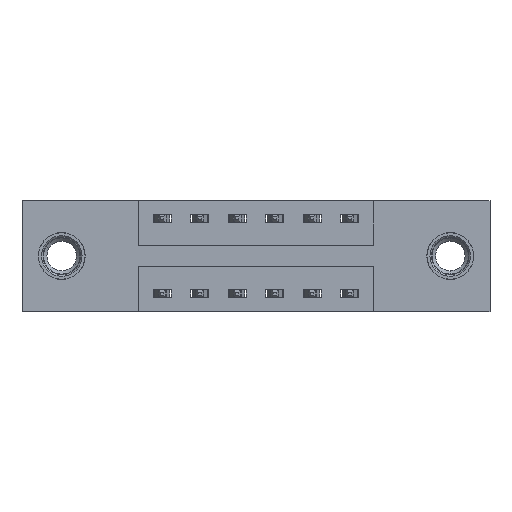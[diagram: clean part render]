
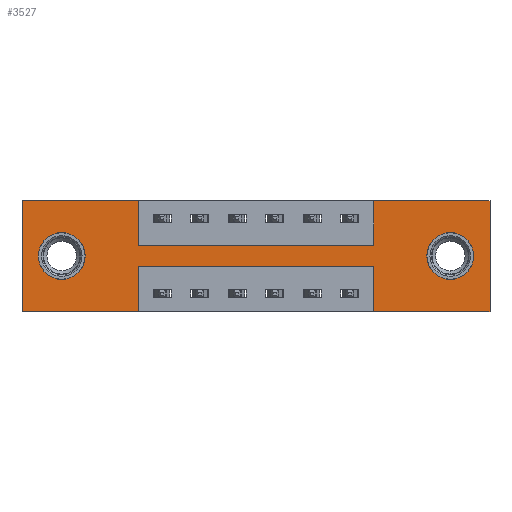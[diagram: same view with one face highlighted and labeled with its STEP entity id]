
A CAD part, front view. The second image highlights one B-rep face of the part: STEP entity #3527.
In plain terms, the highlighted planar face has unit normal (0, -1, 0).
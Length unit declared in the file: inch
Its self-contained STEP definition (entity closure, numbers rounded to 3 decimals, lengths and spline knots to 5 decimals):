
#77 = VECTOR ( 'NONE', #1908, 39.37008 ) ;
#117 = DIRECTION ( 'NONE',  ( 0., 0., -1. ) ) ;
#195 = DIRECTION ( 'NONE',  ( 0., 0., 1. ) ) ;
#220 = DIRECTION ( 'NONE',  ( -1., 0., 0. ) ) ;
#312 = AXIS2_PLACEMENT_3D ( 'NONE', #3044, #5407, #547 ) ;
#351 = CIRCLE ( 'NONE', #3444, 0.078 ) ;
#493 = CARTESIAN_POINT ( 'NONE',  ( 0.3875, 0., -0.22 ) ) ;
#547 = DIRECTION ( 'NONE',  ( 0., 0., -1. ) ) ;
#624 = DIRECTION ( 'NONE',  ( 0., 0., -1. ) ) ;
#731 = EDGE_CURVE ( 'NONE', #2609, #8651, #817, .T. ) ;
#736 = VECTOR ( 'NONE', #195, 39.37008 ) ;
#804 = AXIS2_PLACEMENT_3D ( 'NONE', #1364, #8633, #4704 ) ;
#805 = VECTOR ( 'NONE', #845, 39.37008 ) ;
#817 = CIRCLE ( 'NONE', #7860, 0.078 ) ;
#823 = FACE_OUTER_BOUND ( 'NONE', #9699, .T. ) ;
#845 = DIRECTION ( 'NONE',  ( -1., 0., 0. ) ) ;
#848 = CARTESIAN_POINT ( 'NONE',  ( 0., 0., -0.37 ) ) ;
#890 = ORIENTED_EDGE ( 'NONE', *, *, #5757, .F. ) ;
#955 = ORIENTED_EDGE ( 'NONE', *, *, #1147, .F. ) ;
#975 = DIRECTION ( 'NONE',  ( 0., 0., -1. ) ) ;
#1002 = CARTESIAN_POINT ( 'NONE',  ( 1.56, 0., 0. ) ) ;
#1065 = DIRECTION ( 'NONE',  ( 0., 0., 1. ) ) ;
#1078 = FACE_BOUND ( 'NONE', #9427, .T. ) ;
#1147 = EDGE_CURVE ( 'NONE', #9044, #2476, #7146, .T. ) ;
#1261 = VERTEX_POINT ( 'NONE', #493 ) ;
#1279 = CARTESIAN_POINT ( 'NONE',  ( 0.3875, 0., 0. ) ) ;
#1359 = DIRECTION ( 'NONE',  ( 1., 0., 0. ) ) ;
#1364 = CARTESIAN_POINT ( 'NONE',  ( 0.1325, 0., -0.185 ) ) ;
#1389 = CARTESIAN_POINT ( 'NONE',  ( 0.3875, 0., -0.37 ) ) ;
#1631 = EDGE_CURVE ( 'NONE', #7315, #5923, #5667, .T. ) ;
#1807 = CARTESIAN_POINT ( 'NONE',  ( 0., 0., 0. ) ) ;
#1809 = CARTESIAN_POINT ( 'NONE',  ( 0.1325, 0., -0.107 ) ) ;
#1888 = VECTOR ( 'NONE', #3370, 39.37008 ) ;
#1908 = DIRECTION ( 'NONE',  ( 1., 0., 0. ) ) ;
#1944 = ORIENTED_EDGE ( 'NONE', *, *, #7622, .F. ) ;
#2019 = CIRCLE ( 'NONE', #7383, 0.078 ) ;
#2164 = LINE ( 'NONE', #2536, #1888 ) ;
#2206 = ORIENTED_EDGE ( 'NONE', *, *, #5881, .F. ) ;
#2476 = VERTEX_POINT ( 'NONE', #9174 ) ;
#2500 = CARTESIAN_POINT ( 'NONE',  ( 1.4275, 0., -0.263 ) ) ;
#2536 = CARTESIAN_POINT ( 'NONE',  ( 1.1725, 0., 0. ) ) ;
#2582 = CARTESIAN_POINT ( 'NONE',  ( 0.3875, 0., -0.37 ) ) ;
#2609 = VERTEX_POINT ( 'NONE', #2500 ) ;
#2694 = VERTEX_POINT ( 'NONE', #7252 ) ;
#2952 = EDGE_CURVE ( 'NONE', #3545, #5074, #4079, .T. ) ;
#2973 = LINE ( 'NONE', #1807, #736 ) ;
#3044 = CARTESIAN_POINT ( 'NONE',  ( 0., 0., -0.37 ) ) ;
#3045 = FACE_BOUND ( 'NONE', #9532, .T. ) ;
#3058 = ORIENTED_EDGE ( 'NONE', *, *, #7810, .F. ) ;
#3063 = VERTEX_POINT ( 'NONE', #5595 ) ;
#3093 = LINE ( 'NONE', #4297, #4957 ) ;
#3182 = ORIENTED_EDGE ( 'NONE', *, *, #7800, .T. ) ;
#3248 = CARTESIAN_POINT ( 'NONE',  ( 0.3875, 0., -0.15 ) ) ;
#3370 = DIRECTION ( 'NONE',  ( 0., 0., 1. ) ) ;
#3444 = AXIS2_PLACEMENT_3D ( 'NONE', #9854, #5480, #624 ) ;
#3527 = ADVANCED_FACE ( 'NONE', ( #3045, #1078, #823 ), #7675, .T. ) ;
#3545 = VERTEX_POINT ( 'NONE', #1389 ) ;
#3589 = DIRECTION ( 'NONE',  ( 0., 1., 0. ) ) ;
#3983 = DIRECTION ( 'NONE',  ( 0., 0., -1. ) ) ;
#4008 = DIRECTION ( 'NONE',  ( 0., 1., 0. ) ) ;
#4010 = CARTESIAN_POINT ( 'NONE',  ( 1.4275, 0., -0.185 ) ) ;
#4079 = LINE ( 'NONE', #6899, #5889 ) ;
#4124 = CARTESIAN_POINT ( 'NONE',  ( 0., 0., -0.37 ) ) ;
#4282 = VERTEX_POINT ( 'NONE', #1002 ) ;
#4297 = CARTESIAN_POINT ( 'NONE',  ( 0.3875, 0., 0. ) ) ;
#4342 = EDGE_CURVE ( 'NONE', #2476, #3063, #7254, .T. ) ;
#4484 = VECTOR ( 'NONE', #117, 39.37008 ) ;
#4512 = VECTOR ( 'NONE', #220, 39.37008 ) ;
#4704 = DIRECTION ( 'NONE',  ( 0., 0., 1. ) ) ;
#4725 = LINE ( 'NONE', #2582, #4484 ) ;
#4826 = EDGE_CURVE ( 'NONE', #3063, #1261, #8540, .T. ) ;
#4901 = ORIENTED_EDGE ( 'NONE', *, *, #7726, .F. ) ;
#4957 = VECTOR ( 'NONE', #5092, 39.37008 ) ;
#5046 = CARTESIAN_POINT ( 'NONE',  ( 1.56, 0., 0. ) ) ;
#5074 = VERTEX_POINT ( 'NONE', #4124 ) ;
#5092 = DIRECTION ( 'NONE',  ( 0., 0., -1. ) ) ;
#5159 = ORIENTED_EDGE ( 'NONE', *, *, #5478, .F. ) ;
#5169 = CARTESIAN_POINT ( 'NONE',  ( 1.1725, 0., -0.37 ) ) ;
#5293 = CARTESIAN_POINT ( 'NONE',  ( 1.56, 0., -0.37 ) ) ;
#5407 = DIRECTION ( 'NONE',  ( 0., -1., 0. ) ) ;
#5476 = ORIENTED_EDGE ( 'NONE', *, *, #731, .T. ) ;
#5478 = EDGE_CURVE ( 'NONE', #9726, #9081, #8526, .T. ) ;
#5480 = DIRECTION ( 'NONE',  ( 0., 1., 0. ) ) ;
#5595 = CARTESIAN_POINT ( 'NONE',  ( 1.1725, 0., -0.22 ) ) ;
#5667 = CIRCLE ( 'NONE', #804, 0.078 ) ;
#5731 = VERTEX_POINT ( 'NONE', #3248 ) ;
#5757 = EDGE_CURVE ( 'NONE', #6712, #4282, #6152, .T. ) ;
#5881 = EDGE_CURVE ( 'NONE', #1261, #3545, #4725, .T. ) ;
#5889 = VECTOR ( 'NONE', #7689, 39.37008 ) ;
#5920 = CARTESIAN_POINT ( 'NONE',  ( 0.3875, 0., -0.15 ) ) ;
#5923 = VERTEX_POINT ( 'NONE', #1809 ) ;
#6152 = LINE ( 'NONE', #9318, #8168 ) ;
#6191 = ORIENTED_EDGE ( 'NONE', *, *, #6883, .F. ) ;
#6240 = LINE ( 'NONE', #5920, #77 ) ;
#6410 = CARTESIAN_POINT ( 'NONE',  ( 1.1725, 0., 0. ) ) ;
#6556 = EDGE_CURVE ( 'NONE', #8651, #2609, #351, .T. ) ;
#6712 = VERTEX_POINT ( 'NONE', #6410 ) ;
#6845 = ORIENTED_EDGE ( 'NONE', *, *, #4826, .F. ) ;
#6883 = EDGE_CURVE ( 'NONE', #5074, #9726, #2973, .T. ) ;
#6899 = CARTESIAN_POINT ( 'NONE',  ( 0., 0., -0.37 ) ) ;
#7009 = ORIENTED_EDGE ( 'NONE', *, *, #1631, .T. ) ;
#7053 = LINE ( 'NONE', #5046, #8826 ) ;
#7135 = ORIENTED_EDGE ( 'NONE', *, *, #6556, .T. ) ;
#7146 = LINE ( 'NONE', #848, #805 ) ;
#7252 = CARTESIAN_POINT ( 'NONE',  ( 1.1725, 0., -0.15 ) ) ;
#7254 = LINE ( 'NONE', #5169, #8997 ) ;
#7315 = VERTEX_POINT ( 'NONE', #8386 ) ;
#7349 = ORIENTED_EDGE ( 'NONE', *, *, #2952, .F. ) ;
#7383 = AXIS2_PLACEMENT_3D ( 'NONE', #8181, #3589, #8915 ) ;
#7622 = EDGE_CURVE ( 'NONE', #2694, #6712, #2164, .T. ) ;
#7675 = PLANE ( 'NONE',  #312 ) ;
#7689 = DIRECTION ( 'NONE',  ( -1., 0., 0. ) ) ;
#7726 = EDGE_CURVE ( 'NONE', #9081, #5731, #3093, .T. ) ;
#7800 = EDGE_CURVE ( 'NONE', #5923, #7315, #2019, .T. ) ;
#7810 = EDGE_CURVE ( 'NONE', #5731, #2694, #6240, .T. ) ;
#7860 = AXIS2_PLACEMENT_3D ( 'NONE', #4010, #4008, #3983 ) ;
#8058 = VECTOR ( 'NONE', #1359, 39.37008 ) ;
#8168 = VECTOR ( 'NONE', #8656, 39.37008 ) ;
#8181 = CARTESIAN_POINT ( 'NONE',  ( 0.1325, 0., -0.185 ) ) ;
#8386 = CARTESIAN_POINT ( 'NONE',  ( 0.1325, 0., -0.263 ) ) ;
#8402 = CARTESIAN_POINT ( 'NONE',  ( 0., 0., 0. ) ) ;
#8526 = LINE ( 'NONE', #8402, #8058 ) ;
#8540 = LINE ( 'NONE', #9539, #4512 ) ;
#8633 = DIRECTION ( 'NONE',  ( 0., 1., 0. ) ) ;
#8651 = VERTEX_POINT ( 'NONE', #9415 ) ;
#8656 = DIRECTION ( 'NONE',  ( 1., 0., 0. ) ) ;
#8715 = EDGE_CURVE ( 'NONE', #4282, #9044, #7053, .T. ) ;
#8745 = CARTESIAN_POINT ( 'NONE',  ( 0., 0., 0. ) ) ;
#8826 = VECTOR ( 'NONE', #975, 39.37008 ) ;
#8915 = DIRECTION ( 'NONE',  ( 0., 0., 1. ) ) ;
#8997 = VECTOR ( 'NONE', #1065, 39.37008 ) ;
#9044 = VERTEX_POINT ( 'NONE', #5293 ) ;
#9081 = VERTEX_POINT ( 'NONE', #1279 ) ;
#9174 = CARTESIAN_POINT ( 'NONE',  ( 1.1725, 0., -0.37 ) ) ;
#9293 = ORIENTED_EDGE ( 'NONE', *, *, #4342, .F. ) ;
#9318 = CARTESIAN_POINT ( 'NONE',  ( 0., 0., 0. ) ) ;
#9359 = ORIENTED_EDGE ( 'NONE', *, *, #8715, .F. ) ;
#9415 = CARTESIAN_POINT ( 'NONE',  ( 1.4275, 0., -0.107 ) ) ;
#9427 = EDGE_LOOP ( 'NONE', ( #3182, #7009 ) ) ;
#9532 = EDGE_LOOP ( 'NONE', ( #7135, #5476 ) ) ;
#9539 = CARTESIAN_POINT ( 'NONE',  ( 0.3875, 0., -0.22 ) ) ;
#9699 = EDGE_LOOP ( 'NONE', ( #2206, #6845, #9293, #955, #9359, #890, #1944, #3058, #4901, #5159, #6191, #7349 ) ) ;
#9726 = VERTEX_POINT ( 'NONE', #8745 ) ;
#9854 = CARTESIAN_POINT ( 'NONE',  ( 1.4275, 0., -0.185 ) ) ;
